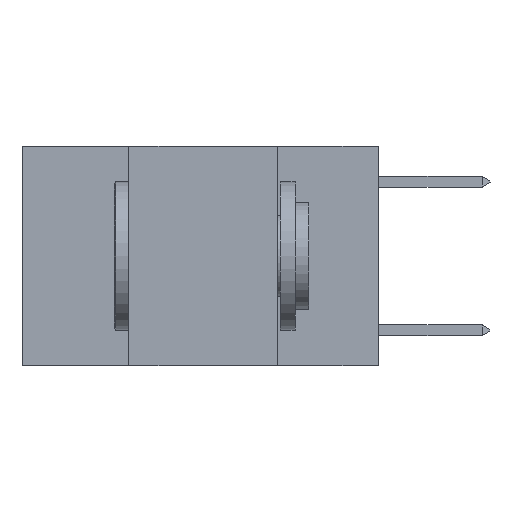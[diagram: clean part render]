
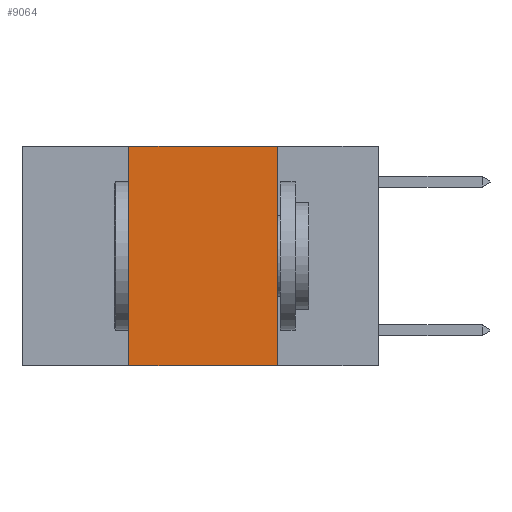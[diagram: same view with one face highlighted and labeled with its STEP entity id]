
A CAD part, left-side view. The second image highlights one B-rep face of the part: STEP entity #9064.
In plain terms, the highlighted planar face has unit normal (-1, 0, 0).
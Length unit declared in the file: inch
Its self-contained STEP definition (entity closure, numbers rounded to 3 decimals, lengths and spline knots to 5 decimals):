
#711 = VERTEX_POINT ( 'NONE', #2412 ) ;
#975 = CARTESIAN_POINT ( 'NONE',  ( 0., 0.42, 0. ) ) ;
#1026 = CARTESIAN_POINT ( 'NONE',  ( 0., 0.17, -0.37 ) ) ;
#1405 = CARTESIAN_POINT ( 'NONE',  ( 0., 0.6, 0. ) ) ;
#1530 = DIRECTION ( 'NONE',  ( 0., 0., -1. ) ) ;
#2016 = CARTESIAN_POINT ( 'NONE',  ( 0., 0.6, -0.37 ) ) ;
#2329 = DIRECTION ( 'NONE',  ( 0., 0., -1. ) ) ;
#2412 = CARTESIAN_POINT ( 'NONE',  ( 0., 0.42, -0.37 ) ) ;
#2612 = EDGE_LOOP ( 'NONE', ( #8308, #6194, #11420, #8269 ) ) ;
#2631 = CARTESIAN_POINT ( 'NONE',  ( 0., 0.6, 0. ) ) ;
#2656 = DIRECTION ( 'NONE',  ( 0., -1., 0. ) ) ;
#2792 = EDGE_CURVE ( 'NONE', #7292, #4039, #3715, .T. ) ;
#3098 = EDGE_CURVE ( 'NONE', #711, #7292, #9099, .T. ) ;
#3169 = CARTESIAN_POINT ( 'NONE',  ( 0., 0.42, 0. ) ) ;
#3715 = LINE ( 'NONE', #2631, #10722 ) ;
#3965 = VECTOR ( 'NONE', #1530, 39.37008 ) ;
#4039 = VERTEX_POINT ( 'NONE', #8945 ) ;
#5108 = EDGE_CURVE ( 'NONE', #4039, #10150, #10971, .T. ) ;
#5328 = VECTOR ( 'NONE', #7499, 39.37008 ) ;
#5998 = PLANE ( 'NONE',  #7560 ) ;
#6194 = ORIENTED_EDGE ( 'NONE', *, *, #2792, .F. ) ;
#6691 = VECTOR ( 'NONE', #9250, 39.37008 ) ;
#7058 = CARTESIAN_POINT ( 'NONE',  ( 0., 0.17, 0. ) ) ;
#7292 = VERTEX_POINT ( 'NONE', #3169 ) ;
#7499 = DIRECTION ( 'NONE',  ( 0., -1., 0. ) ) ;
#7560 = AXIS2_PLACEMENT_3D ( 'NONE', #1405, #7821, #2329 ) ;
#7821 = DIRECTION ( 'NONE',  ( 1., 0., 0. ) ) ;
#8269 = ORIENTED_EDGE ( 'NONE', *, *, #8393, .T. ) ;
#8308 = ORIENTED_EDGE ( 'NONE', *, *, #5108, .F. ) ;
#8393 = EDGE_CURVE ( 'NONE', #711, #10150, #10166, .T. ) ;
#8945 = CARTESIAN_POINT ( 'NONE',  ( 0., 0.17, 0. ) ) ;
#9064 = ADVANCED_FACE ( 'NONE', ( #11725 ), #5998, .F. ) ;
#9099 = LINE ( 'NONE', #975, #6691 ) ;
#9250 = DIRECTION ( 'NONE',  ( 0., 0., 1. ) ) ;
#10150 = VERTEX_POINT ( 'NONE', #1026 ) ;
#10166 = LINE ( 'NONE', #2016, #5328 ) ;
#10722 = VECTOR ( 'NONE', #2656, 39.37008 ) ;
#10971 = LINE ( 'NONE', #7058, #3965 ) ;
#11420 = ORIENTED_EDGE ( 'NONE', *, *, #3098, .F. ) ;
#11725 = FACE_OUTER_BOUND ( 'NONE', #2612, .T. ) ;
